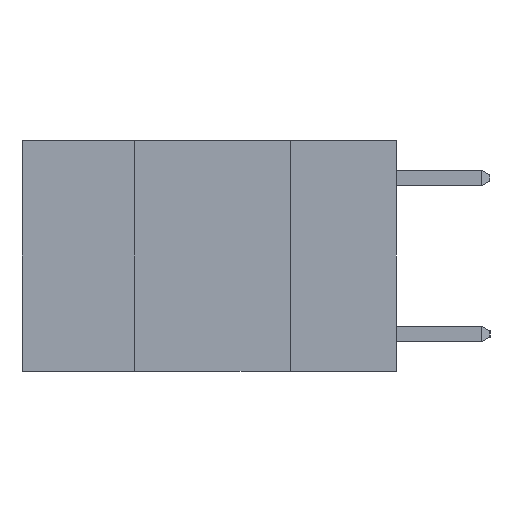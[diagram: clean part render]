
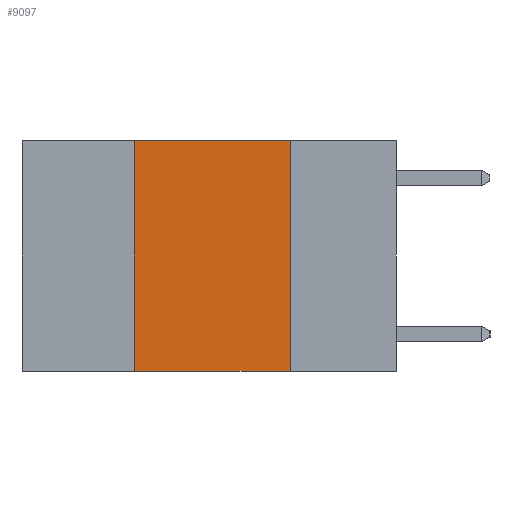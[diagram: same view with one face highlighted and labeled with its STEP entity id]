
A CAD part, left-side view. The second image highlights one B-rep face of the part: STEP entity #9097.
In plain terms, the highlighted planar face has unit normal (-1, 0, 0).
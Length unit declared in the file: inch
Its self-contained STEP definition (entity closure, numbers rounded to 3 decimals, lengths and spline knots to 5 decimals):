
#255 = DIRECTION ( 'NONE',  ( 0., -1., 0. ) ) ;
#427 = VECTOR ( 'NONE', #5126, 39.37008 ) ;
#486 = DIRECTION ( 'NONE',  ( 0., 0., 1. ) ) ;
#682 = EDGE_CURVE ( 'NONE', #4982, #10154, #5057, .T. ) ;
#1517 = FACE_OUTER_BOUND ( 'NONE', #3040, .T. ) ;
#1652 = CARTESIAN_POINT ( 'NONE',  ( 0., 0.6, 0. ) ) ;
#2310 = VECTOR ( 'NONE', #255, 39.37008 ) ;
#2477 = EDGE_CURVE ( 'NONE', #10154, #4514, #7593, .T. ) ;
#2771 = EDGE_CURVE ( 'NONE', #5571, #4514, #4754, .T. ) ;
#3040 = EDGE_LOOP ( 'NONE', ( #8589, #4755, #6075, #8554 ) ) ;
#4514 = VERTEX_POINT ( 'NONE', #8491 ) ;
#4754 = LINE ( 'NONE', #7692, #2310 ) ;
#4755 = ORIENTED_EDGE ( 'NONE', *, *, #682, .F. ) ;
#4982 = VERTEX_POINT ( 'NONE', #7187 ) ;
#5057 = LINE ( 'NONE', #1652, #427 ) ;
#5126 = DIRECTION ( 'NONE',  ( 0., -1., 0. ) ) ;
#5144 = LINE ( 'NONE', #10394, #10084 ) ;
#5549 = CARTESIAN_POINT ( 'NONE',  ( 0., 0.17, 0. ) ) ;
#5571 = VERTEX_POINT ( 'NONE', #7919 ) ;
#5742 = DIRECTION ( 'NONE',  ( 0., 0., -1. ) ) ;
#6075 = ORIENTED_EDGE ( 'NONE', *, *, #8138, .F. ) ;
#6492 = DIRECTION ( 'NONE',  ( 0., 0., -1. ) ) ;
#7187 = CARTESIAN_POINT ( 'NONE',  ( 0., 0.42, 0. ) ) ;
#7331 = VECTOR ( 'NONE', #6492, 39.37008 ) ;
#7593 = LINE ( 'NONE', #9815, #7331 ) ;
#7692 = CARTESIAN_POINT ( 'NONE',  ( 0., 0.6, -0.37 ) ) ;
#7919 = CARTESIAN_POINT ( 'NONE',  ( 0., 0.42, -0.37 ) ) ;
#8138 = EDGE_CURVE ( 'NONE', #5571, #4982, #5144, .T. ) ;
#8230 = CARTESIAN_POINT ( 'NONE',  ( 0., 0.6, 0. ) ) ;
#8491 = CARTESIAN_POINT ( 'NONE',  ( 0., 0.17, -0.37 ) ) ;
#8554 = ORIENTED_EDGE ( 'NONE', *, *, #2771, .T. ) ;
#8589 = ORIENTED_EDGE ( 'NONE', *, *, #2477, .F. ) ;
#9068 = DIRECTION ( 'NONE',  ( 1., 0., 0. ) ) ;
#9097 = ADVANCED_FACE ( 'NONE', ( #1517 ), #9903, .F. ) ;
#9815 = CARTESIAN_POINT ( 'NONE',  ( 0., 0.17, 0. ) ) ;
#9903 = PLANE ( 'NONE',  #10276 ) ;
#10084 = VECTOR ( 'NONE', #486, 39.37008 ) ;
#10154 = VERTEX_POINT ( 'NONE', #5549 ) ;
#10276 = AXIS2_PLACEMENT_3D ( 'NONE', #8230, #9068, #5742 ) ;
#10394 = CARTESIAN_POINT ( 'NONE',  ( 0., 0.42, 0. ) ) ;
